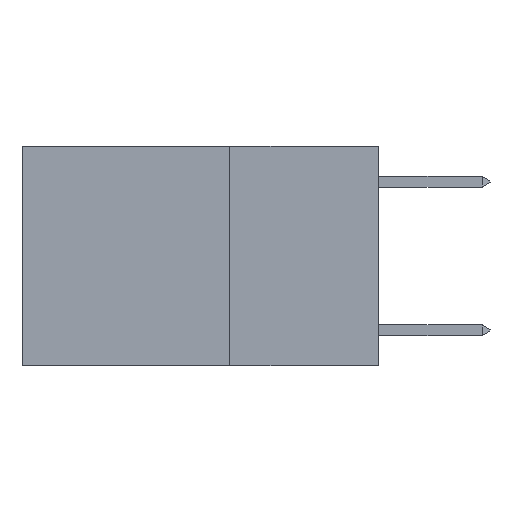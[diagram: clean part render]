
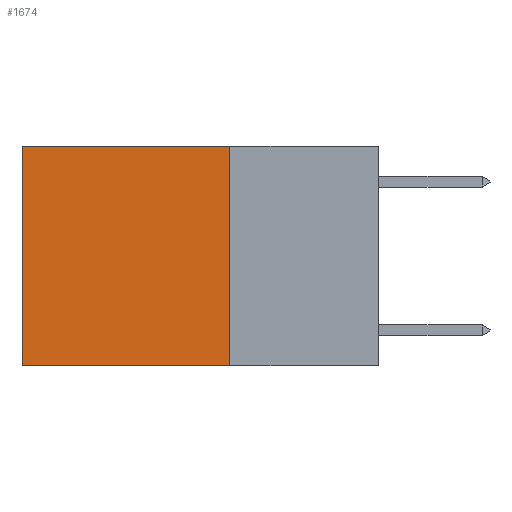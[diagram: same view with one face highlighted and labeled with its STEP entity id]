
A CAD part, left-side view. The second image highlights one B-rep face of the part: STEP entity #1674.
In plain terms, the highlighted planar face has unit normal (-1, 0, 0).
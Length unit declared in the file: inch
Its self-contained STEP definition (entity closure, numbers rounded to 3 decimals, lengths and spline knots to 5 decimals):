
#843 = DIRECTION ( 'NONE',  ( 0., 0., -1. ) ) ;
#1080 = PLANE ( 'NONE',  #8099 ) ;
#1390 = ORIENTED_EDGE ( 'NONE', *, *, #6949, .T. ) ;
#1456 = CARTESIAN_POINT ( 'NONE',  ( 0.2625, 0.25, 0. ) ) ;
#1521 = ORIENTED_EDGE ( 'NONE', *, *, #5290, .F. ) ;
#1674 = ADVANCED_FACE ( 'NONE', ( #12422 ), #1080, .F. ) ;
#1836 = VECTOR ( 'NONE', #13699, 39.37008 ) ;
#2351 = VECTOR ( 'NONE', #13947, 39.37008 ) ;
#2669 = DIRECTION ( 'NONE',  ( 0., 0., -1. ) ) ;
#2919 = EDGE_CURVE ( 'NONE', #7969, #12963, #14225, .T. ) ;
#5112 = VECTOR ( 'NONE', #8702, 39.37008 ) ;
#5290 = EDGE_CURVE ( 'NONE', #12963, #8753, #8280, .T. ) ;
#5481 = VERTEX_POINT ( 'NONE', #11600 ) ;
#5624 = DIRECTION ( 'NONE',  ( 1., 0., 0. ) ) ;
#5664 = ORIENTED_EDGE ( 'NONE', *, *, #2919, .F. ) ;
#5791 = CARTESIAN_POINT ( 'NONE',  ( 0.2625, 0.25, -0.37 ) ) ;
#6818 = CARTESIAN_POINT ( 'NONE',  ( 0.2625, 0.25, 0. ) ) ;
#6949 = EDGE_CURVE ( 'NONE', #5481, #8753, #14089, .T. ) ;
#7388 = CARTESIAN_POINT ( 'NONE',  ( 0.2625, 0.6, 0. ) ) ;
#7546 = CARTESIAN_POINT ( 'NONE',  ( 0.2625, 0.25, 0. ) ) ;
#7969 = VERTEX_POINT ( 'NONE', #7546 ) ;
#8099 = AXIS2_PLACEMENT_3D ( 'NONE', #6818, #5624, #843 ) ;
#8280 = LINE ( 'NONE', #9403, #2351 ) ;
#8702 = DIRECTION ( 'NONE',  ( 0., 0., -1. ) ) ;
#8753 = VERTEX_POINT ( 'NONE', #9160 ) ;
#8912 = ORIENTED_EDGE ( 'NONE', *, *, #13067, .T. ) ;
#9160 = CARTESIAN_POINT ( 'NONE',  ( 0.2625, 0.6, -0.37 ) ) ;
#9403 = CARTESIAN_POINT ( 'NONE',  ( 0.2625, 0.25, -0.37 ) ) ;
#10086 = VECTOR ( 'NONE', #2669, 39.37008 ) ;
#10853 = EDGE_LOOP ( 'NONE', ( #1390, #1521, #5664, #8912 ) ) ;
#11600 = CARTESIAN_POINT ( 'NONE',  ( 0.2625, 0.6, 0. ) ) ;
#12422 = FACE_OUTER_BOUND ( 'NONE', #10853, .T. ) ;
#12805 = LINE ( 'NONE', #1456, #1836 ) ;
#12963 = VERTEX_POINT ( 'NONE', #5791 ) ;
#13067 = EDGE_CURVE ( 'NONE', #7969, #5481, #12805, .T. ) ;
#13699 = DIRECTION ( 'NONE',  ( 0., 1., 0. ) ) ;
#13947 = DIRECTION ( 'NONE',  ( 0., 1., 0. ) ) ;
#14089 = LINE ( 'NONE', #7388, #10086 ) ;
#14225 = LINE ( 'NONE', #14521, #5112 ) ;
#14521 = CARTESIAN_POINT ( 'NONE',  ( 0.2625, 0.25, 0. ) ) ;
